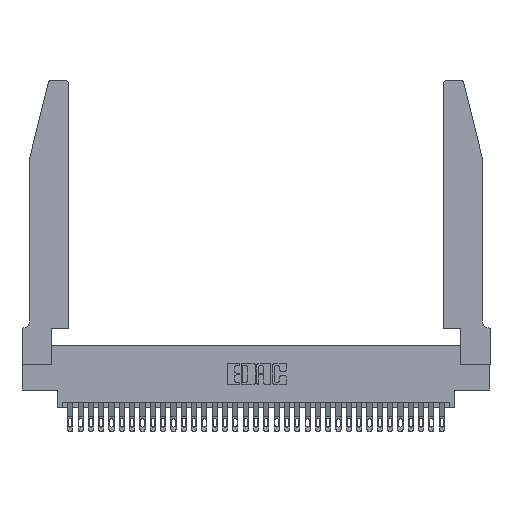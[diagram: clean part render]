
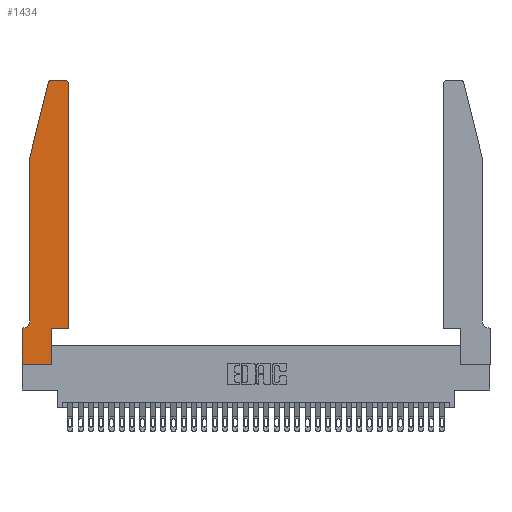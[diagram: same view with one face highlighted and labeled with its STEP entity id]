
A CAD part, top view. The second image highlights one B-rep face of the part: STEP entity #1434.
In plain terms, the highlighted planar face has unit normal (0, 0, 1).
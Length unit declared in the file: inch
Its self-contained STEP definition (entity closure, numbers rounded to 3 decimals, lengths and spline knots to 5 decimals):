
#174 = VECTOR ( 'NONE', #25751, 39.37008 ) ;
#460 = VECTOR ( 'NONE', #5009, 39.37008 ) ;
#1203 = CIRCLE ( 'NONE', #6707, 0.07 ) ;
#1228 = CARTESIAN_POINT ( 'NONE',  ( 0., 0.35, 0.37 ) ) ;
#1372 = CARTESIAN_POINT ( 'NONE',  ( 0., 0., 0.37 ) ) ;
#1434 = ADVANCED_FACE ( 'NONE', ( #26515 ), #25476, .T. ) ;
#1997 = EDGE_CURVE ( 'NONE', #30863, #12163, #32732, .T. ) ;
#2797 = EDGE_CURVE ( 'NONE', #7484, #18406, #8271, .T. ) ;
#3243 = VERTEX_POINT ( 'NONE', #13968 ) ;
#3267 = AXIS2_PLACEMENT_3D ( 'NONE', #1228, #6711, #25595 ) ;
#3488 = ORIENTED_EDGE ( 'NONE', *, *, #1997, .T. ) ;
#3577 = DIRECTION ( 'NONE',  ( 0., 0., 1. ) ) ;
#3658 = CARTESIAN_POINT ( 'NONE',  ( 0.0755, 2., 0.37 ) ) ;
#4000 = DIRECTION ( 'NONE',  ( -1., 0., 0. ) ) ;
#4051 = EDGE_CURVE ( 'NONE', #27006, #13090, #5026, .T. ) ;
#4817 = CARTESIAN_POINT ( 'NONE',  ( 0.4205, 2.75, 0.37 ) ) ;
#5009 = DIRECTION ( 'NONE',  ( 0., 1., 0. ) ) ;
#5026 = LINE ( 'NONE', #12132, #18563 ) ;
#5276 = ORIENTED_EDGE ( 'NONE', *, *, #29859, .T. ) ;
#6355 = EDGE_CURVE ( 'NONE', #3243, #15033, #33474, .T. ) ;
#6402 = DIRECTION ( 'NONE',  ( 0., -1., 0. ) ) ;
#6649 = EDGE_CURVE ( 'NONE', #12163, #3243, #32221, .T. ) ;
#6707 = AXIS2_PLACEMENT_3D ( 'NONE', #9731, #28580, #12480 ) ;
#6711 = DIRECTION ( 'NONE',  ( 0., 0., 1. ) ) ;
#6756 = CARTESIAN_POINT ( 'NONE',  ( 0.4205, 2.72, 0.37 ) ) ;
#6824 = CARTESIAN_POINT ( 'NONE',  ( 0.2865, 0.35, 0.37 ) ) ;
#7160 = VERTEX_POINT ( 'NONE', #4817 ) ;
#7410 = ORIENTED_EDGE ( 'NONE', *, *, #6649, .T. ) ;
#7484 = VERTEX_POINT ( 'NONE', #27673 ) ;
#7573 = CARTESIAN_POINT ( 'NONE',  ( 0.0755, 2., 0.37 ) ) ;
#7815 = ORIENTED_EDGE ( 'NONE', *, *, #30363, .T. ) ;
#7930 = CARTESIAN_POINT ( 'NONE',  ( 0.0755, 0.42, 0.37 ) ) ;
#8271 = LINE ( 'NONE', #1372, #174 ) ;
#8721 = ORIENTED_EDGE ( 'NONE', *, *, #31177, .T. ) ;
#9192 = VECTOR ( 'NONE', #18777, 39.37008 ) ;
#9459 = DIRECTION ( 'NONE',  ( 1., 0., 0. ) ) ;
#9731 = CARTESIAN_POINT ( 'NONE',  ( 0.0055, 0.42, 0.37 ) ) ;
#10043 = LINE ( 'NONE', #13369, #9192 ) ;
#10066 = EDGE_CURVE ( 'NONE', #15163, #7160, #19458, .T. ) ;
#10570 = CARTESIAN_POINT ( 'NONE',  ( 0.0055, 0.35, 0.37 ) ) ;
#12132 = CARTESIAN_POINT ( 'NONE',  ( 0.4505, 0.35, 0.37 ) ) ;
#12163 = VERTEX_POINT ( 'NONE', #18569 ) ;
#12480 = DIRECTION ( 'NONE',  ( -1., 0., 0. ) ) ;
#13090 = VERTEX_POINT ( 'NONE', #14284 ) ;
#13369 = CARTESIAN_POINT ( 'NONE',  ( 0., 0., 0.37 ) ) ;
#13781 = VECTOR ( 'NONE', #6402, 39.37008 ) ;
#13885 = EDGE_CURVE ( 'NONE', #7160, #30863, #14695, .T. ) ;
#13968 = CARTESIAN_POINT ( 'NONE',  ( 0.0755, 2., 0.37 ) ) ;
#14210 = ORIENTED_EDGE ( 'NONE', *, *, #10066, .T. ) ;
#14284 = CARTESIAN_POINT ( 'NONE',  ( 0.4505, 0.35, 0.37 ) ) ;
#14695 = LINE ( 'NONE', #26999, #21019 ) ;
#14770 = LINE ( 'NONE', #22914, #20249 ) ;
#14836 = DIRECTION ( 'NONE',  ( 1., 0., 0. ) ) ;
#14904 = CARTESIAN_POINT ( 'NONE',  ( 0.284, 2.75, 0.37 ) ) ;
#15033 = VERTEX_POINT ( 'NONE', #7930 ) ;
#15163 = VERTEX_POINT ( 'NONE', #16460 ) ;
#15878 = CARTESIAN_POINT ( 'NONE',  ( 0., 0.35, 0.37 ) ) ;
#16460 = CARTESIAN_POINT ( 'NONE',  ( 0.4505, 2.72, 0.37 ) ) ;
#18255 = ORIENTED_EDGE ( 'NONE', *, *, #18320, .T. ) ;
#18320 = EDGE_CURVE ( 'NONE', #18406, #27006, #22088, .T. ) ;
#18406 = VERTEX_POINT ( 'NONE', #24961 ) ;
#18563 = VECTOR ( 'NONE', #14836, 39.37008 ) ;
#18569 = CARTESIAN_POINT ( 'NONE',  ( 0.25487, 2.72718, 0.37 ) ) ;
#18777 = DIRECTION ( 'NONE',  ( 0., -1., 0. ) ) ;
#19449 = DIRECTION ( 'NONE',  ( 0., 1., 0. ) ) ;
#19458 = CIRCLE ( 'NONE', #30986, 0.03 ) ;
#19813 = CARTESIAN_POINT ( 'NONE',  ( 0.284, 2.72, 0.37 ) ) ;
#20249 = VECTOR ( 'NONE', #4000, 39.37008 ) ;
#20727 = AXIS2_PLACEMENT_3D ( 'NONE', #19813, #3577, #22506 ) ;
#21019 = VECTOR ( 'NONE', #27112, 39.37008 ) ;
#22088 = LINE ( 'NONE', #26489, #460 ) ;
#22506 = DIRECTION ( 'NONE',  ( 1., 0., 0. ) ) ;
#22914 = CARTESIAN_POINT ( 'NONE',  ( 0.0755, 0.35, 0.37 ) ) ;
#23509 = VERTEX_POINT ( 'NONE', #10570 ) ;
#24770 = ORIENTED_EDGE ( 'NONE', *, *, #6355, .T. ) ;
#24961 = CARTESIAN_POINT ( 'NONE',  ( 0.2865, 0., 0.37 ) ) ;
#25217 = ORIENTED_EDGE ( 'NONE', *, *, #29583, .T. ) ;
#25476 = PLANE ( 'NONE',  #3267 ) ;
#25595 = DIRECTION ( 'NONE',  ( 1., 0., 0. ) ) ;
#25643 = DIRECTION ( 'NONE',  ( 0., 0., 1. ) ) ;
#25751 = DIRECTION ( 'NONE',  ( 1., 0., 0. ) ) ;
#26489 = CARTESIAN_POINT ( 'NONE',  ( 0.2865, 0.35, 0.37 ) ) ;
#26515 = FACE_OUTER_BOUND ( 'NONE', #31993, .T. ) ;
#26563 = VERTEX_POINT ( 'NONE', #15878 ) ;
#26999 = CARTESIAN_POINT ( 'NONE',  ( 0.2605, 2.75, 0.37 ) ) ;
#27006 = VERTEX_POINT ( 'NONE', #6824 ) ;
#27112 = DIRECTION ( 'NONE',  ( -1., 0., 0. ) ) ;
#27536 = ORIENTED_EDGE ( 'NONE', *, *, #4051, .T. ) ;
#27673 = CARTESIAN_POINT ( 'NONE',  ( 0., 0., 0.37 ) ) ;
#28580 = DIRECTION ( 'NONE',  ( 0., 0., -1. ) ) ;
#29583 = EDGE_CURVE ( 'NONE', #13090, #15163, #31970, .T. ) ;
#29859 = EDGE_CURVE ( 'NONE', #15033, #23509, #1203, .T. ) ;
#30363 = EDGE_CURVE ( 'NONE', #23509, #26563, #14770, .T. ) ;
#30863 = VERTEX_POINT ( 'NONE', #14904 ) ;
#30986 = AXIS2_PLACEMENT_3D ( 'NONE', #6756, #25643, #9459 ) ;
#31177 = EDGE_CURVE ( 'NONE', #26563, #7484, #10043, .T. ) ;
#31386 = VECTOR ( 'NONE', #31701, 39.37008 ) ;
#31701 = DIRECTION ( 'NONE',  ( -0.239, -0.971, 0. ) ) ;
#31970 = LINE ( 'NONE', #32549, #34729 ) ;
#31993 = EDGE_LOOP ( 'NONE', ( #34614, #3488, #7410, #24770, #5276, #7815, #8721, #34130, #18255, #27536, #25217, #14210 ) ) ;
#32221 = LINE ( 'NONE', #7573, #31386 ) ;
#32549 = CARTESIAN_POINT ( 'NONE',  ( 0.4505, 0.35, 0.37 ) ) ;
#32732 = CIRCLE ( 'NONE', #20727, 0.03 ) ;
#33474 = LINE ( 'NONE', #3658, #13781 ) ;
#34130 = ORIENTED_EDGE ( 'NONE', *, *, #2797, .T. ) ;
#34614 = ORIENTED_EDGE ( 'NONE', *, *, #13885, .T. ) ;
#34729 = VECTOR ( 'NONE', #19449, 39.37008 ) ;
